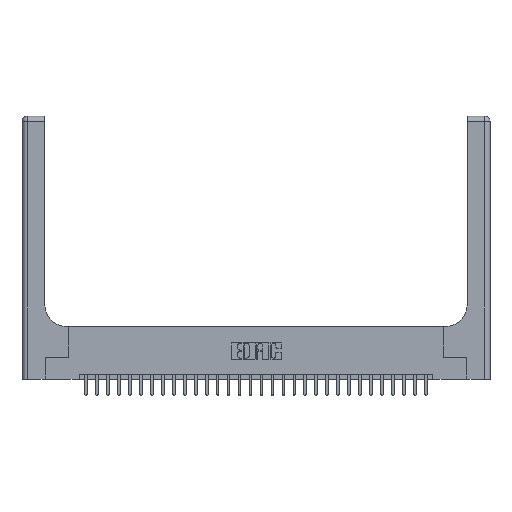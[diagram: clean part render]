
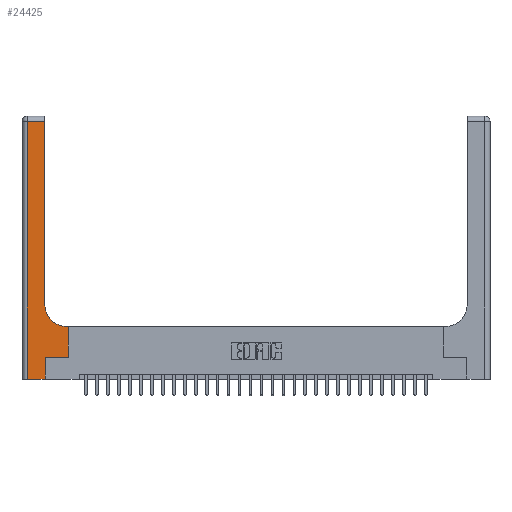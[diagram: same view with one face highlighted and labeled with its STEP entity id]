
A CAD part, top view. The second image highlights one B-rep face of the part: STEP entity #24425.
In plain terms, the highlighted planar face has unit normal (0, 0, 1).
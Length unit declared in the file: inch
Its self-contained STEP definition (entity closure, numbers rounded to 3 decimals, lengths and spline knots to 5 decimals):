
#848 = PLANE ( 'NONE',  #9527 ) ;
#2043 = LINE ( 'NONE', #27391, #24095 ) ;
#2669 = DIRECTION ( 'NONE',  ( 1., 0., 0. ) ) ;
#2686 = VERTEX_POINT ( 'NONE', #19180 ) ;
#2768 = VERTEX_POINT ( 'NONE', #22395 ) ;
#2843 = EDGE_CURVE ( 'NONE', #25361, #26488, #26343, .T. ) ;
#2858 = VERTEX_POINT ( 'NONE', #13851 ) ;
#3976 = LINE ( 'NONE', #21906, #12350 ) ;
#4585 = DIRECTION ( 'NONE',  ( 1., 0., 0. ) ) ;
#4781 = LINE ( 'NONE', #9743, #5454 ) ;
#5454 = VECTOR ( 'NONE', #12190, 39.37008 ) ;
#5470 = ORIENTED_EDGE ( 'NONE', *, *, #2843, .T. ) ;
#7140 = EDGE_CURVE ( 'NONE', #15656, #14621, #23056, .T. ) ;
#7319 = ORIENTED_EDGE ( 'NONE', *, *, #7976, .T. ) ;
#7350 = CARTESIAN_POINT ( 'NONE',  ( 0., 3., 0.37 ) ) ;
#7976 = EDGE_CURVE ( 'NONE', #25126, #2768, #25368, .T. ) ;
#8001 = CARTESIAN_POINT ( 'NONE',  ( 0.06, 0., 0.37 ) ) ;
#8101 = DIRECTION ( 'NONE',  ( 0., 1., 0. ) ) ;
#8364 = CARTESIAN_POINT ( 'NONE',  ( 0.26, 2.94, 0.37 ) ) ;
#8509 = DIRECTION ( 'NONE',  ( 0., -1., 0. ) ) ;
#8731 = FACE_OUTER_BOUND ( 'NONE', #9427, .T. ) ;
#9427 = EDGE_LOOP ( 'NONE', ( #5470, #23651, #24524, #16355, #24354, #7319, #10081, #25192, #10102 ) ) ;
#9527 = AXIS2_PLACEMENT_3D ( 'NONE', #7350, #15693, #22286 ) ;
#9743 = CARTESIAN_POINT ( 'NONE',  ( 0., 2.94, 0.37 ) ) ;
#10081 = ORIENTED_EDGE ( 'NONE', *, *, #17191, .T. ) ;
#10102 = ORIENTED_EDGE ( 'NONE', *, *, #10962, .T. ) ;
#10962 = EDGE_CURVE ( 'NONE', #12605, #25361, #19766, .T. ) ;
#11707 = DIRECTION ( 'NONE',  ( 0., 1., 0. ) ) ;
#11783 = EDGE_CURVE ( 'NONE', #14621, #2686, #3976, .T. ) ;
#12190 = DIRECTION ( 'NONE',  ( -1., 0., 0. ) ) ;
#12350 = VECTOR ( 'NONE', #24087, 39.37008 ) ;
#12605 = VERTEX_POINT ( 'NONE', #26027 ) ;
#13262 = CARTESIAN_POINT ( 'NONE',  ( 0.06, 2.94, 0.37 ) ) ;
#13587 = EDGE_CURVE ( 'NONE', #2686, #25126, #17090, .T. ) ;
#13619 = CARTESIAN_POINT ( 'NONE',  ( 0.265, 0.25, 0.37 ) ) ;
#13752 = CARTESIAN_POINT ( 'NONE',  ( 0.26, 3., 0.37 ) ) ;
#13851 = CARTESIAN_POINT ( 'NONE',  ( 0.528, 0.6, 0.37 ) ) ;
#14621 = VERTEX_POINT ( 'NONE', #8001 ) ;
#14722 = VECTOR ( 'NONE', #15285, 39.37008 ) ;
#15285 = DIRECTION ( 'NONE',  ( -1., 0., 0. ) ) ;
#15656 = VERTEX_POINT ( 'NONE', #13262 ) ;
#15693 = DIRECTION ( 'NONE',  ( 0., 0., -1. ) ) ;
#15884 = CARTESIAN_POINT ( 'NONE',  ( 0.265, 0., 0.37 ) ) ;
#16282 = AXIS2_PLACEMENT_3D ( 'NONE', #19167, #23652, #4585 ) ;
#16355 = ORIENTED_EDGE ( 'NONE', *, *, #11783, .T. ) ;
#16447 = CARTESIAN_POINT ( 'NONE',  ( 0.06, 3., 0.37 ) ) ;
#17090 = LINE ( 'NONE', #15884, #23571 ) ;
#17191 = EDGE_CURVE ( 'NONE', #2768, #2858, #2043, .T. ) ;
#18022 = LINE ( 'NONE', #25465, #14722 ) ;
#18343 = CARTESIAN_POINT ( 'NONE',  ( 0.26, 0.85, 0.37 ) ) ;
#19167 = CARTESIAN_POINT ( 'NONE',  ( 0.51, 0.85, 0.37 ) ) ;
#19180 = CARTESIAN_POINT ( 'NONE',  ( 0.265, 0., 0.37 ) ) ;
#19766 = CIRCLE ( 'NONE', #16282, 0.25 ) ;
#20165 = EDGE_CURVE ( 'NONE', #26488, #15656, #4781, .T. ) ;
#20642 = VECTOR ( 'NONE', #11707, 39.37008 ) ;
#21324 = VECTOR ( 'NONE', #2669, 39.37008 ) ;
#21450 = DIRECTION ( 'NONE',  ( 0., 1., 0. ) ) ;
#21906 = CARTESIAN_POINT ( 'NONE',  ( 0., 0., 0.37 ) ) ;
#22155 = CARTESIAN_POINT ( 'NONE',  ( 0.265, 0.25, 0.37 ) ) ;
#22286 = DIRECTION ( 'NONE',  ( -1., 0., 0. ) ) ;
#22395 = CARTESIAN_POINT ( 'NONE',  ( 0.528, 0.25, 0.37 ) ) ;
#23056 = LINE ( 'NONE', #16447, #24414 ) ;
#23571 = VECTOR ( 'NONE', #21450, 39.37008 ) ;
#23634 = EDGE_CURVE ( 'NONE', #2858, #12605, #18022, .T. ) ;
#23651 = ORIENTED_EDGE ( 'NONE', *, *, #20165, .T. ) ;
#23652 = DIRECTION ( 'NONE',  ( 0., 0., -1. ) ) ;
#24087 = DIRECTION ( 'NONE',  ( 1., 0., 0. ) ) ;
#24095 = VECTOR ( 'NONE', #8101, 39.37008 ) ;
#24354 = ORIENTED_EDGE ( 'NONE', *, *, #13587, .T. ) ;
#24414 = VECTOR ( 'NONE', #8509, 39.37008 ) ;
#24425 = ADVANCED_FACE ( 'NONE', ( #8731 ), #848, .F. ) ;
#24524 = ORIENTED_EDGE ( 'NONE', *, *, #7140, .T. ) ;
#25126 = VERTEX_POINT ( 'NONE', #22155 ) ;
#25192 = ORIENTED_EDGE ( 'NONE', *, *, #23634, .T. ) ;
#25361 = VERTEX_POINT ( 'NONE', #18343 ) ;
#25368 = LINE ( 'NONE', #13619, #21324 ) ;
#25465 = CARTESIAN_POINT ( 'NONE',  ( 0.26, 0.6, 0.37 ) ) ;
#26027 = CARTESIAN_POINT ( 'NONE',  ( 0.51, 0.6, 0.37 ) ) ;
#26343 = LINE ( 'NONE', #13752, #20642 ) ;
#26488 = VERTEX_POINT ( 'NONE', #8364 ) ;
#27391 = CARTESIAN_POINT ( 'NONE',  ( 0.528, 0.25, 0.37 ) ) ;
